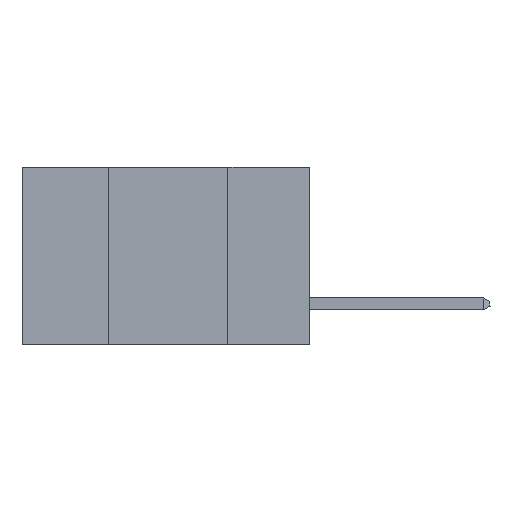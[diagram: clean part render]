
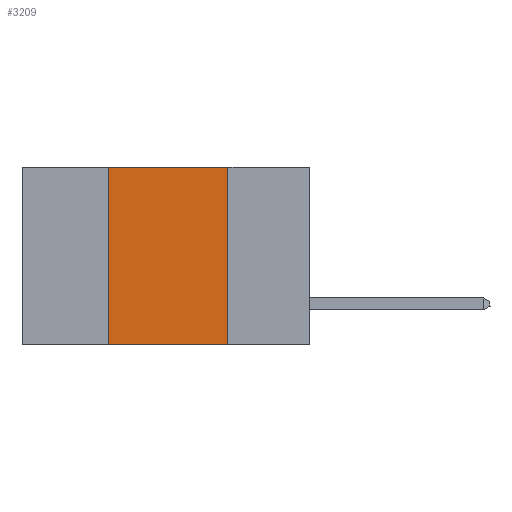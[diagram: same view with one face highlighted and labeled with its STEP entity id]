
A CAD part, left-side view. The second image highlights one B-rep face of the part: STEP entity #3209.
In plain terms, the highlighted planar face has unit normal (-1, 0, 0).
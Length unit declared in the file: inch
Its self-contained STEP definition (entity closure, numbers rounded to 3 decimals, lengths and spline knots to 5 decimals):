
#451 = CARTESIAN_POINT ( 'NONE',  ( 0., 0.42, 0. ) ) ;
#1097 = DIRECTION ( 'NONE',  ( 0., 0., 1. ) ) ;
#1286 = EDGE_LOOP ( 'NONE', ( #2875, #12915, #13868, #20889 ) ) ;
#1352 = VECTOR ( 'NONE', #1097, 39.37008 ) ;
#1961 = VERTEX_POINT ( 'NONE', #31037 ) ;
#2875 = ORIENTED_EDGE ( 'NONE', *, *, #17197, .F. ) ;
#3209 = ADVANCED_FACE ( 'NONE', ( #3966 ), #21329, .F. ) ;
#3614 = CARTESIAN_POINT ( 'NONE',  ( 0., 0.6, -0.37 ) ) ;
#3966 = FACE_OUTER_BOUND ( 'NONE', #1286, .T. ) ;
#4101 = DIRECTION ( 'NONE',  ( 0., 0., -1. ) ) ;
#5190 = VECTOR ( 'NONE', #4101, 39.37008 ) ;
#7892 = DIRECTION ( 'NONE',  ( 1., 0., 0. ) ) ;
#8106 = VERTEX_POINT ( 'NONE', #33869 ) ;
#8503 = CARTESIAN_POINT ( 'NONE',  ( 0., 0.42, -0.37 ) ) ;
#9365 = CARTESIAN_POINT ( 'NONE',  ( 0., 0.17, 0. ) ) ;
#9927 = LINE ( 'NONE', #9365, #5190 ) ;
#10504 = EDGE_CURVE ( 'NONE', #1961, #8106, #21596, .T. ) ;
#12915 = ORIENTED_EDGE ( 'NONE', *, *, #10504, .F. ) ;
#13009 = LINE ( 'NONE', #451, #1352 ) ;
#13868 = ORIENTED_EDGE ( 'NONE', *, *, #16505, .F. ) ;
#13929 = EDGE_CURVE ( 'NONE', #25686, #31337, #33620, .T. ) ;
#16143 = CARTESIAN_POINT ( 'NONE',  ( 0., 0.6, 0. ) ) ;
#16487 = CARTESIAN_POINT ( 'NONE',  ( 0., 0.17, -0.37 ) ) ;
#16505 = EDGE_CURVE ( 'NONE', #25686, #1961, #13009, .T. ) ;
#17197 = EDGE_CURVE ( 'NONE', #8106, #31337, #9927, .T. ) ;
#20889 = ORIENTED_EDGE ( 'NONE', *, *, #13929, .T. ) ;
#21329 = PLANE ( 'NONE',  #28603 ) ;
#21596 = LINE ( 'NONE', #16143, #33940 ) ;
#22947 = VECTOR ( 'NONE', #25584, 39.37008 ) ;
#24233 = CARTESIAN_POINT ( 'NONE',  ( 0., 0.6, 0. ) ) ;
#24451 = DIRECTION ( 'NONE',  ( 0., 0., -1. ) ) ;
#25584 = DIRECTION ( 'NONE',  ( 0., -1., 0. ) ) ;
#25686 = VERTEX_POINT ( 'NONE', #8503 ) ;
#28603 = AXIS2_PLACEMENT_3D ( 'NONE', #24233, #7892, #24451 ) ;
#29527 = DIRECTION ( 'NONE',  ( 0., -1., 0. ) ) ;
#31037 = CARTESIAN_POINT ( 'NONE',  ( 0., 0.42, 0. ) ) ;
#31337 = VERTEX_POINT ( 'NONE', #16487 ) ;
#33620 = LINE ( 'NONE', #3614, #22947 ) ;
#33869 = CARTESIAN_POINT ( 'NONE',  ( 0., 0.17, 0. ) ) ;
#33940 = VECTOR ( 'NONE', #29527, 39.37008 ) ;
